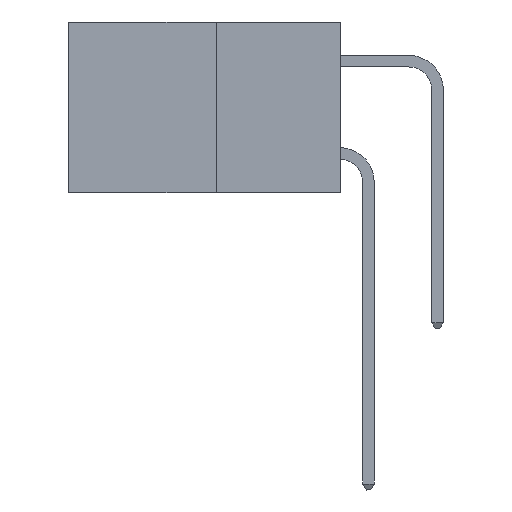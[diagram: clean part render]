
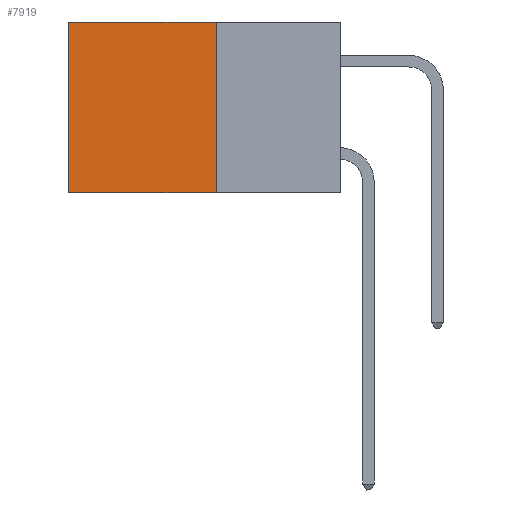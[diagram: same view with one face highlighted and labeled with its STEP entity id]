
A CAD part, left-side view. The second image highlights one B-rep face of the part: STEP entity #7919.
In plain terms, the highlighted planar face has unit normal (-1, 0, 0).
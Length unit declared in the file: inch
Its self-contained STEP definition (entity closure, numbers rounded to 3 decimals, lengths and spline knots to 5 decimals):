
#571 = ORIENTED_EDGE ( 'NONE', *, *, #15278, .T. ) ;
#1793 = LINE ( 'NONE', #5617, #28007 ) ;
#2848 = PLANE ( 'NONE',  #16690 ) ;
#5525 = DIRECTION ( 'NONE',  ( 1., 0., 0. ) ) ;
#5617 = CARTESIAN_POINT ( 'NONE',  ( 0.277, 0.27, 0. ) ) ;
#5973 = LINE ( 'NONE', #29393, #12197 ) ;
#6085 = EDGE_CURVE ( 'NONE', #12206, #25179, #5973, .T. ) ;
#6322 = EDGE_CURVE ( 'NONE', #13605, #26603, #18714, .T. ) ;
#6577 = CARTESIAN_POINT ( 'NONE',  ( 0.277, 0.27, -0.37 ) ) ;
#7919 = ADVANCED_FACE ( 'NONE', ( #25094 ), #2848, .F. ) ;
#9261 = DIRECTION ( 'NONE',  ( 0., 1., 0. ) ) ;
#11317 = DIRECTION ( 'NONE',  ( 0., 0., -1. ) ) ;
#12197 = VECTOR ( 'NONE', #11317, 39.37008 ) ;
#12206 = VERTEX_POINT ( 'NONE', #21244 ) ;
#12213 = DIRECTION ( 'NONE',  ( 0., 0., -1. ) ) ;
#13605 = VERTEX_POINT ( 'NONE', #19815 ) ;
#15278 = EDGE_CURVE ( 'NONE', #13605, #12206, #1793, .T. ) ;
#15297 = CARTESIAN_POINT ( 'NONE',  ( 0.277, 0.27, -0.37 ) ) ;
#16426 = VECTOR ( 'NONE', #9261, 39.37008 ) ;
#16604 = ORIENTED_EDGE ( 'NONE', *, *, #6322, .F. ) ;
#16690 = AXIS2_PLACEMENT_3D ( 'NONE', #18508, #5525, #23838 ) ;
#18016 = CARTESIAN_POINT ( 'NONE',  ( 0.277, 0.59, -0.37 ) ) ;
#18508 = CARTESIAN_POINT ( 'NONE',  ( 0.277, 0.27, -0.37 ) ) ;
#18714 = LINE ( 'NONE', #30390, #32522 ) ;
#19815 = CARTESIAN_POINT ( 'NONE',  ( 0.277, 0.27, 0. ) ) ;
#21244 = CARTESIAN_POINT ( 'NONE',  ( 0.277, 0.59, 0. ) ) ;
#23838 = DIRECTION ( 'NONE',  ( 0., 0., -1. ) ) ;
#23895 = EDGE_LOOP ( 'NONE', ( #24913, #30973, #16604, #571 ) ) ;
#24140 = LINE ( 'NONE', #6577, #16426 ) ;
#24913 = ORIENTED_EDGE ( 'NONE', *, *, #6085, .T. ) ;
#25094 = FACE_OUTER_BOUND ( 'NONE', #23895, .T. ) ;
#25179 = VERTEX_POINT ( 'NONE', #18016 ) ;
#26603 = VERTEX_POINT ( 'NONE', #15297 ) ;
#28007 = VECTOR ( 'NONE', #31658, 39.37008 ) ;
#28365 = EDGE_CURVE ( 'NONE', #26603, #25179, #24140, .T. ) ;
#29393 = CARTESIAN_POINT ( 'NONE',  ( 0.277, 0.59, -0.37 ) ) ;
#30390 = CARTESIAN_POINT ( 'NONE',  ( 0.277, 0.27, -0.37 ) ) ;
#30973 = ORIENTED_EDGE ( 'NONE', *, *, #28365, .F. ) ;
#31658 = DIRECTION ( 'NONE',  ( 0., 1., 0. ) ) ;
#32522 = VECTOR ( 'NONE', #12213, 39.37008 ) ;
